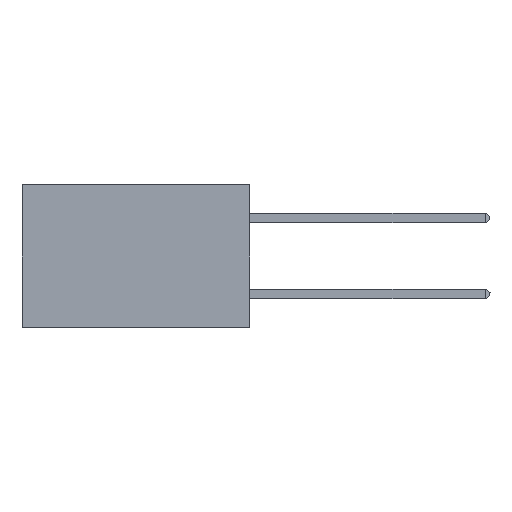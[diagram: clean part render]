
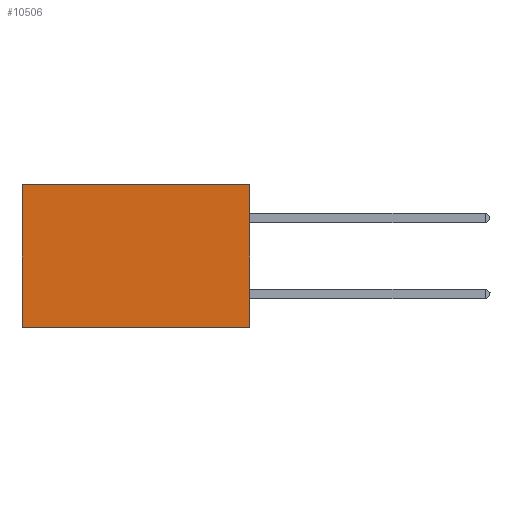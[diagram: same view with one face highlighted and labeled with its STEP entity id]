
A CAD part, left-side view. The second image highlights one B-rep face of the part: STEP entity #10506.
In plain terms, the highlighted planar face has unit normal (-1, 0, 0).
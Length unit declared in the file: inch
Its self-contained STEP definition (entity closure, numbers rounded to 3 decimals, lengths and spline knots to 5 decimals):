
#163 = AXIS2_PLACEMENT_3D ( 'NONE', #3696, #10882, #14493 ) ;
#832 = CARTESIAN_POINT ( 'NONE',  ( 0.2875, 0.6, -0.375 ) ) ;
#901 = EDGE_LOOP ( 'NONE', ( #13907, #5709, #9905, #7850 ) ) ;
#1147 = LINE ( 'NONE', #12203, #14972 ) ;
#1173 = LINE ( 'NONE', #8840, #4678 ) ;
#3157 = EDGE_CURVE ( 'NONE', #8196, #13749, #1147, .T. ) ;
#3696 = CARTESIAN_POINT ( 'NONE',  ( 0.2875, 0., -0.375 ) ) ;
#3905 = VECTOR ( 'NONE', #8568, 39.37008 ) ;
#4678 = VECTOR ( 'NONE', #5426, 39.37008 ) ;
#5426 = DIRECTION ( 'NONE',  ( 0., 1., 0. ) ) ;
#5508 = VECTOR ( 'NONE', #13810, 39.37008 ) ;
#5709 = ORIENTED_EDGE ( 'NONE', *, *, #6644, .F. ) ;
#6101 = PLANE ( 'NONE',  #163 ) ;
#6268 = LINE ( 'NONE', #832, #5508 ) ;
#6644 = EDGE_CURVE ( 'NONE', #13749, #10444, #1173, .T. ) ;
#7557 = FACE_OUTER_BOUND ( 'NONE', #901, .T. ) ;
#7850 = ORIENTED_EDGE ( 'NONE', *, *, #8952, .T. ) ;
#8196 = VERTEX_POINT ( 'NONE', #11619 ) ;
#8568 = DIRECTION ( 'NONE',  ( 0., 1., 0. ) ) ;
#8840 = CARTESIAN_POINT ( 'NONE',  ( 0.2875, 0., -0.375 ) ) ;
#8952 = EDGE_CURVE ( 'NONE', #8196, #12908, #13230, .T. ) ;
#9905 = ORIENTED_EDGE ( 'NONE', *, *, #3157, .F. ) ;
#9932 = CARTESIAN_POINT ( 'NONE',  ( 0.2875, 0., 0. ) ) ;
#10444 = VERTEX_POINT ( 'NONE', #15139 ) ;
#10506 = ADVANCED_FACE ( 'NONE', ( #7557 ), #6101, .F. ) ;
#10882 = DIRECTION ( 'NONE',  ( 1., 0., 0. ) ) ;
#11619 = CARTESIAN_POINT ( 'NONE',  ( 0.2875, 0., 0. ) ) ;
#12108 = EDGE_CURVE ( 'NONE', #12908, #10444, #6268, .T. ) ;
#12203 = CARTESIAN_POINT ( 'NONE',  ( 0.2875, 0., -0.375 ) ) ;
#12908 = VERTEX_POINT ( 'NONE', #14719 ) ;
#13230 = LINE ( 'NONE', #9932, #3905 ) ;
#13749 = VERTEX_POINT ( 'NONE', #14976 ) ;
#13810 = DIRECTION ( 'NONE',  ( 0., 0., -1. ) ) ;
#13907 = ORIENTED_EDGE ( 'NONE', *, *, #12108, .T. ) ;
#14493 = DIRECTION ( 'NONE',  ( 0., 0., -1. ) ) ;
#14719 = CARTESIAN_POINT ( 'NONE',  ( 0.2875, 0.6, 0. ) ) ;
#14749 = DIRECTION ( 'NONE',  ( 0., 0., -1. ) ) ;
#14972 = VECTOR ( 'NONE', #14749, 39.37008 ) ;
#14976 = CARTESIAN_POINT ( 'NONE',  ( 0.2875, 0., -0.375 ) ) ;
#15139 = CARTESIAN_POINT ( 'NONE',  ( 0.2875, 0.6, -0.375 ) ) ;
